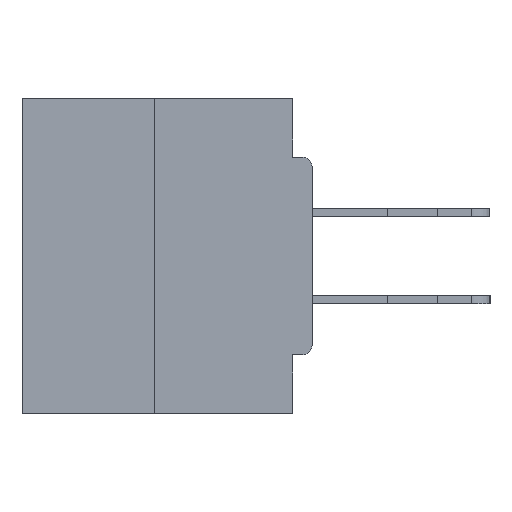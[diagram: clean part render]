
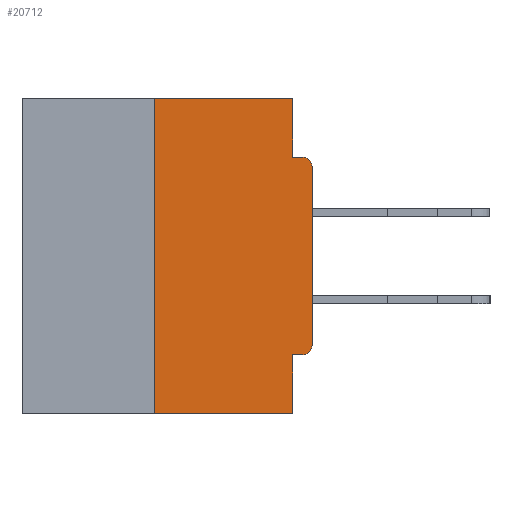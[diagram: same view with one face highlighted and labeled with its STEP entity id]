
A CAD part, left-side view. The second image highlights one B-rep face of the part: STEP entity #20712.
In plain terms, the highlighted planar face has unit normal (-1, 0, 0).
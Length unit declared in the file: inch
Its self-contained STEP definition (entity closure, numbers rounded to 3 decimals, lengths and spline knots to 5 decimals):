
#863 = ORIENTED_EDGE ( 'NONE', *, *, #19008, .F. ) ;
#1488 = VERTEX_POINT ( 'NONE', #14168 ) ;
#1572 = VECTOR ( 'NONE', #29848, 39.37008 ) ;
#2119 = EDGE_LOOP ( 'NONE', ( #10989, #27371, #7299, #863, #17531, #26339, #26914, #26899, #10610, #6886 ) ) ;
#3347 = CARTESIAN_POINT ( 'NONE',  ( 0., 0.25, 0. ) ) ;
#3932 = CARTESIAN_POINT ( 'NONE',  ( 0., 0.46, -0.5 ) ) ;
#4176 = DIRECTION ( 'NONE',  ( 0., 0., 1. ) ) ;
#4374 = DIRECTION ( 'NONE',  ( 0., -1., 0. ) ) ;
#4450 = VECTOR ( 'NONE', #4374, 39.37008 ) ;
#4968 = CARTESIAN_POINT ( 'NONE',  ( 0., 0.031, 0. ) ) ;
#6210 = CARTESIAN_POINT ( 'NONE',  ( 0., 0.015, -0.0935 ) ) ;
#6270 = EDGE_CURVE ( 'NONE', #27349, #7425, #23864, .T. ) ;
#6298 = CARTESIAN_POINT ( 'NONE',  ( 0., 0.031, -0.5 ) ) ;
#6603 = DIRECTION ( 'NONE',  ( -1., 0., 0. ) ) ;
#6629 = CARTESIAN_POINT ( 'NONE',  ( 0., 0.031, -0.4065 ) ) ;
#6886 = ORIENTED_EDGE ( 'NONE', *, *, #28392, .F. ) ;
#7146 = LINE ( 'NONE', #4968, #29459 ) ;
#7253 = DIRECTION ( 'NONE',  ( 0., 0., -1. ) ) ;
#7299 = ORIENTED_EDGE ( 'NONE', *, *, #14286, .T. ) ;
#7425 = VERTEX_POINT ( 'NONE', #6629 ) ;
#7476 = DIRECTION ( 'NONE',  ( 1., 0., 0. ) ) ;
#7539 = DIRECTION ( 'NONE',  ( 0., -1., 0. ) ) ;
#7699 = CARTESIAN_POINT ( 'NONE',  ( 0., 0.031, -0.5 ) ) ;
#8434 = CARTESIAN_POINT ( 'NONE',  ( 0., 0.015, -0.4065 ) ) ;
#8616 = FACE_OUTER_BOUND ( 'NONE', #2119, .T. ) ;
#8649 = EDGE_CURVE ( 'NONE', #27926, #26585, #15198, .T. ) ;
#9077 = VERTEX_POINT ( 'NONE', #14299 ) ;
#9183 = CIRCLE ( 'NONE', #14601, 0.015 ) ;
#9271 = CARTESIAN_POINT ( 'NONE',  ( 0., 0., -0.4065 ) ) ;
#10401 = EDGE_CURVE ( 'NONE', #1488, #9077, #17412, .T. ) ;
#10610 = ORIENTED_EDGE ( 'NONE', *, *, #25489, .F. ) ;
#10782 = AXIS2_PLACEMENT_3D ( 'NONE', #27412, #7476, #7253 ) ;
#10989 = ORIENTED_EDGE ( 'NONE', *, *, #8649, .F. ) ;
#11075 = VECTOR ( 'NONE', #4176, 39.37008 ) ;
#11237 = DIRECTION ( 'NONE',  ( 0., -1., 0. ) ) ;
#12269 = EDGE_CURVE ( 'NONE', #28717, #27926, #26904, .T. ) ;
#12566 = DIRECTION ( 'NONE',  ( 0., 0., -1. ) ) ;
#13701 = CARTESIAN_POINT ( 'NONE',  ( 0., 0., -0.0935 ) ) ;
#14168 = CARTESIAN_POINT ( 'NONE',  ( 0., 0., -0.3915 ) ) ;
#14286 = EDGE_CURVE ( 'NONE', #28717, #32713, #22757, .T. ) ;
#14299 = CARTESIAN_POINT ( 'NONE',  ( 0., 0., -0.1085 ) ) ;
#14601 = AXIS2_PLACEMENT_3D ( 'NONE', #29310, #6603, #23956 ) ;
#15198 = LINE ( 'NONE', #17769, #19921 ) ;
#17412 = LINE ( 'NONE', #26984, #11075 ) ;
#17531 = ORIENTED_EDGE ( 'NONE', *, *, #6270, .F. ) ;
#17769 = CARTESIAN_POINT ( 'NONE',  ( 0., 0.46, 0. ) ) ;
#17833 = DIRECTION ( 'NONE',  ( 0., 0., -1. ) ) ;
#18371 = CIRCLE ( 'NONE', #18894, 0.015 ) ;
#18685 = EDGE_CURVE ( 'NONE', #27349, #1488, #9183, .T. ) ;
#18780 = CARTESIAN_POINT ( 'NONE',  ( 0., 0.015, -0.1085 ) ) ;
#18894 = AXIS2_PLACEMENT_3D ( 'NONE', #18780, #21303, #21647 ) ;
#19008 = EDGE_CURVE ( 'NONE', #7425, #32713, #24253, .T. ) ;
#19738 = VECTOR ( 'NONE', #29085, 39.37008 ) ;
#19921 = VECTOR ( 'NONE', #7539, 39.37008 ) ;
#20685 = CARTESIAN_POINT ( 'NONE',  ( 0., 0.031, 0. ) ) ;
#20712 = ADVANCED_FACE ( 'NONE', ( #8616 ), #22270, .F. ) ;
#21303 = DIRECTION ( 'NONE',  ( -1., 0., 0. ) ) ;
#21647 = DIRECTION ( 'NONE',  ( 0., 0., -1. ) ) ;
#22270 = PLANE ( 'NONE',  #10782 ) ;
#22581 = CARTESIAN_POINT ( 'NONE',  ( 0., 0.031, -0.0935 ) ) ;
#22757 = LINE ( 'NONE', #3932, #4450 ) ;
#23164 = LINE ( 'NONE', #13701, #31556 ) ;
#23864 = LINE ( 'NONE', #9271, #1572 ) ;
#23956 = DIRECTION ( 'NONE',  ( 0., 0., -1. ) ) ;
#24253 = LINE ( 'NONE', #7699, #29447 ) ;
#25395 = EDGE_CURVE ( 'NONE', #9077, #25468, #18371, .T. ) ;
#25468 = VERTEX_POINT ( 'NONE', #6210 ) ;
#25489 = EDGE_CURVE ( 'NONE', #27794, #25468, #23164, .T. ) ;
#26323 = CARTESIAN_POINT ( 'NONE',  ( 0., 0.25, -0.5 ) ) ;
#26339 = ORIENTED_EDGE ( 'NONE', *, *, #18685, .T. ) ;
#26585 = VERTEX_POINT ( 'NONE', #20685 ) ;
#26899 = ORIENTED_EDGE ( 'NONE', *, *, #25395, .T. ) ;
#26904 = LINE ( 'NONE', #3347, #19738 ) ;
#26914 = ORIENTED_EDGE ( 'NONE', *, *, #10401, .T. ) ;
#26984 = CARTESIAN_POINT ( 'NONE',  ( 0., 0., 0. ) ) ;
#27349 = VERTEX_POINT ( 'NONE', #8434 ) ;
#27371 = ORIENTED_EDGE ( 'NONE', *, *, #12269, .F. ) ;
#27412 = CARTESIAN_POINT ( 'NONE',  ( 0., 0.46, 0. ) ) ;
#27794 = VERTEX_POINT ( 'NONE', #22581 ) ;
#27926 = VERTEX_POINT ( 'NONE', #28498 ) ;
#28392 = EDGE_CURVE ( 'NONE', #26585, #27794, #7146, .T. ) ;
#28498 = CARTESIAN_POINT ( 'NONE',  ( 0., 0.25, 0. ) ) ;
#28717 = VERTEX_POINT ( 'NONE', #26323 ) ;
#29085 = DIRECTION ( 'NONE',  ( 0., 0., 1. ) ) ;
#29310 = CARTESIAN_POINT ( 'NONE',  ( 0., 0.015, -0.3915 ) ) ;
#29447 = VECTOR ( 'NONE', #17833, 39.37008 ) ;
#29459 = VECTOR ( 'NONE', #12566, 39.37008 ) ;
#29848 = DIRECTION ( 'NONE',  ( 0., 1., 0. ) ) ;
#31556 = VECTOR ( 'NONE', #11237, 39.37008 ) ;
#32713 = VERTEX_POINT ( 'NONE', #6298 ) ;
